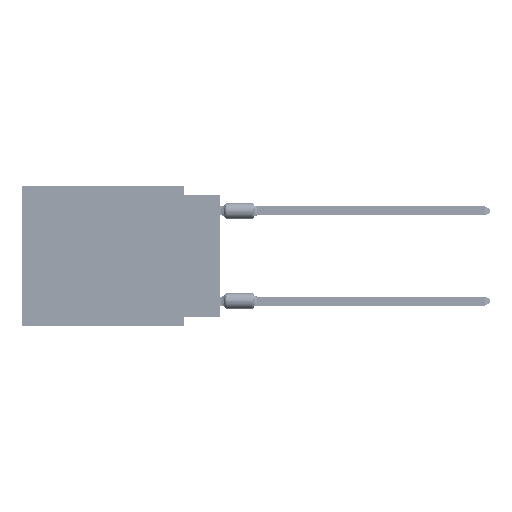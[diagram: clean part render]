
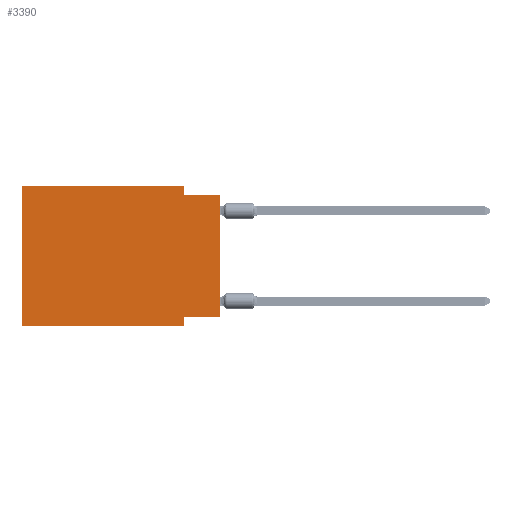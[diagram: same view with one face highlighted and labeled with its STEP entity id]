
A CAD part, left-side view. The second image highlights one B-rep face of the part: STEP entity #3390.
In plain terms, the highlighted planar face has unit normal (-1, 0, 0).
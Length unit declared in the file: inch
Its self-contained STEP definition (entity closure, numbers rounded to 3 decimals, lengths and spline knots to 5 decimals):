
#1056 = EDGE_CURVE ( 'NONE', #19226, #10165, #10330, .T. ) ;
#1941 = CARTESIAN_POINT ( 'NONE',  ( 0., 0.1, -0.39 ) ) ;
#2103 = CARTESIAN_POINT ( 'NONE',  ( 0., 0.55, -0.39 ) ) ;
#2686 = CARTESIAN_POINT ( 'NONE',  ( 0., 0.55, 0. ) ) ;
#3339 = CARTESIAN_POINT ( 'NONE',  ( 0., 0.1, -0.39 ) ) ;
#3390 = ADVANCED_FACE ( 'NONE', ( #51048 ), #55940, .F. ) ;
#3415 = CARTESIAN_POINT ( 'NONE',  ( 0., 0., -0.025 ) ) ;
#4412 = VECTOR ( 'NONE', #50140, 39.37008 ) ;
#5786 = CARTESIAN_POINT ( 'NONE',  ( 0., 0., 0. ) ) ;
#6160 = EDGE_CURVE ( 'NONE', #19226, #34149, #65691, .T. ) ;
#6238 = EDGE_LOOP ( 'NONE', ( #49051, #46260, #35041, #34208, #26890, #53704, #37790, #38319 ) ) ;
#7736 = DIRECTION ( 'NONE',  ( 0., 0., -1. ) ) ;
#10165 = VERTEX_POINT ( 'NONE', #54195 ) ;
#10330 = LINE ( 'NONE', #5786, #42032 ) ;
#11345 = DIRECTION ( 'NONE',  ( 0., 0., -1. ) ) ;
#11797 = AXIS2_PLACEMENT_3D ( 'NONE', #29054, #66754, #7736 ) ;
#13719 = VECTOR ( 'NONE', #59097, 39.37008 ) ;
#14020 = EDGE_CURVE ( 'NONE', #53591, #10165, #20163, .T. ) ;
#15791 = CARTESIAN_POINT ( 'NONE',  ( 0., 0.55, 0. ) ) ;
#15934 = EDGE_CURVE ( 'NONE', #37468, #53591, #59189, .T. ) ;
#17828 = CARTESIAN_POINT ( 'NONE',  ( 0., 0., -0.365 ) ) ;
#19226 = VERTEX_POINT ( 'NONE', #17828 ) ;
#19933 = VECTOR ( 'NONE', #30987, 39.37008 ) ;
#20163 = LINE ( 'NONE', #3415, #19933 ) ;
#20901 = CARTESIAN_POINT ( 'NONE',  ( 0., 0.55, -0.39 ) ) ;
#21373 = LINE ( 'NONE', #15791, #26864 ) ;
#22076 = EDGE_CURVE ( 'NONE', #46119, #37468, #44831, .T. ) ;
#23424 = VECTOR ( 'NONE', #11345, 39.37008 ) ;
#25789 = DIRECTION ( 'NONE',  ( 0., -1., 0. ) ) ;
#26044 = EDGE_CURVE ( 'NONE', #41431, #46119, #21373, .T. ) ;
#26835 = LINE ( 'NONE', #20901, #42411 ) ;
#26864 = VECTOR ( 'NONE', #32196, 39.37008 ) ;
#26890 = ORIENTED_EDGE ( 'NONE', *, *, #26044, .F. ) ;
#29054 = CARTESIAN_POINT ( 'NONE',  ( 0., 0.55, 0. ) ) ;
#30987 = DIRECTION ( 'NONE',  ( 0., -1., 0. ) ) ;
#31266 = CARTESIAN_POINT ( 'NONE',  ( 0., 0.1, 0. ) ) ;
#32196 = DIRECTION ( 'NONE',  ( 0., 0., 1. ) ) ;
#34149 = VERTEX_POINT ( 'NONE', #55341 ) ;
#34208 = ORIENTED_EDGE ( 'NONE', *, *, #22076, .F. ) ;
#35041 = ORIENTED_EDGE ( 'NONE', *, *, #15934, .F. ) ;
#37468 = VERTEX_POINT ( 'NONE', #38550 ) ;
#37790 = ORIENTED_EDGE ( 'NONE', *, *, #48791, .F. ) ;
#38319 = ORIENTED_EDGE ( 'NONE', *, *, #6160, .F. ) ;
#38550 = CARTESIAN_POINT ( 'NONE',  ( 0., 0.1, 0. ) ) ;
#41431 = VERTEX_POINT ( 'NONE', #2103 ) ;
#42032 = VECTOR ( 'NONE', #63416, 39.37008 ) ;
#42411 = VECTOR ( 'NONE', #25789, 39.37008 ) ;
#44831 = LINE ( 'NONE', #45526, #52139 ) ;
#45526 = CARTESIAN_POINT ( 'NONE',  ( 0., 0.55, 0. ) ) ;
#45819 = EDGE_CURVE ( 'NONE', #41431, #62259, #26835, .T. ) ;
#46119 = VERTEX_POINT ( 'NONE', #2686 ) ;
#46260 = ORIENTED_EDGE ( 'NONE', *, *, #14020, .F. ) ;
#48310 = CARTESIAN_POINT ( 'NONE',  ( 0., 0., -0.365 ) ) ;
#48791 = EDGE_CURVE ( 'NONE', #34149, #62259, #49122, .T. ) ;
#49051 = ORIENTED_EDGE ( 'NONE', *, *, #1056, .T. ) ;
#49122 = LINE ( 'NONE', #1941, #4412 ) ;
#50140 = DIRECTION ( 'NONE',  ( 0., 0., -1. ) ) ;
#50336 = CARTESIAN_POINT ( 'NONE',  ( 0., 0.1, -0.025 ) ) ;
#51048 = FACE_OUTER_BOUND ( 'NONE', #6238, .T. ) ;
#51086 = DIRECTION ( 'NONE',  ( 0., -1., 0. ) ) ;
#52139 = VECTOR ( 'NONE', #51086, 39.37008 ) ;
#53591 = VERTEX_POINT ( 'NONE', #50336 ) ;
#53704 = ORIENTED_EDGE ( 'NONE', *, *, #45819, .T. ) ;
#54195 = CARTESIAN_POINT ( 'NONE',  ( 0., 0., -0.025 ) ) ;
#55341 = CARTESIAN_POINT ( 'NONE',  ( 0., 0.1, -0.365 ) ) ;
#55940 = PLANE ( 'NONE',  #11797 ) ;
#59097 = DIRECTION ( 'NONE',  ( 0., 1., 0. ) ) ;
#59189 = LINE ( 'NONE', #31266, #23424 ) ;
#62259 = VERTEX_POINT ( 'NONE', #3339 ) ;
#63416 = DIRECTION ( 'NONE',  ( 0., 0., 1. ) ) ;
#65691 = LINE ( 'NONE', #48310, #13719 ) ;
#66754 = DIRECTION ( 'NONE',  ( 1., 0., 0. ) ) ;
